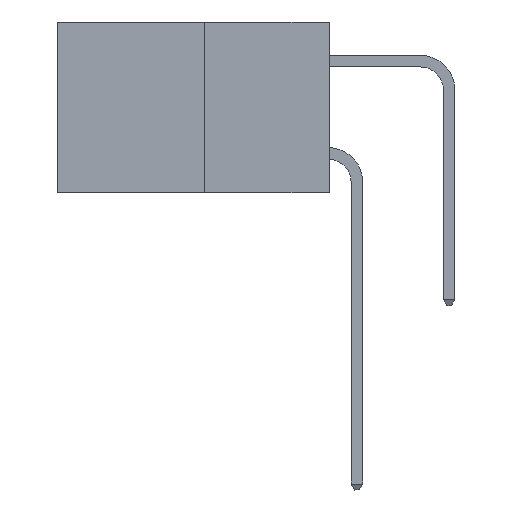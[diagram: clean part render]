
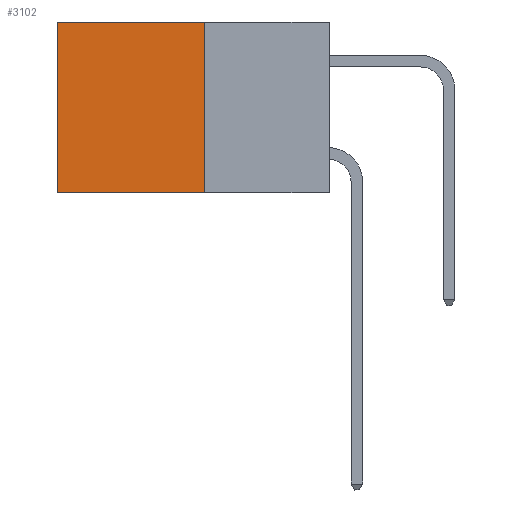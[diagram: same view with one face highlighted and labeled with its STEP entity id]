
A CAD part, left-side view. The second image highlights one B-rep face of the part: STEP entity #3102.
In plain terms, the highlighted planar face has unit normal (-1, 0, 0).
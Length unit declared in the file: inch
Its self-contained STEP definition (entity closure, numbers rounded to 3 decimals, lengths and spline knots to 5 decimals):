
#769 = CARTESIAN_POINT ( 'NONE',  ( 0.277, 0.27, -0.37 ) ) ;
#1806 = EDGE_CURVE ( 'NONE', #21932, #14569, #10224, .T. ) ;
#1830 = CARTESIAN_POINT ( 'NONE',  ( 0.277, 0.59, -0.37 ) ) ;
#2989 = EDGE_CURVE ( 'NONE', #21932, #9261, #9326, .T. ) ;
#3102 = ADVANCED_FACE ( 'NONE', ( #20293 ), #15326, .F. ) ;
#3221 = LINE ( 'NONE', #1830, #3775 ) ;
#3611 = DIRECTION ( 'NONE',  ( 0., 0., -1. ) ) ;
#3775 = VECTOR ( 'NONE', #3611, 39.37008 ) ;
#4475 = DIRECTION ( 'NONE',  ( 0., 0., -1. ) ) ;
#5391 = DIRECTION ( 'NONE',  ( 0., 0., -1. ) ) ;
#5444 = CARTESIAN_POINT ( 'NONE',  ( 0.277, 0.27, -0.37 ) ) ;
#5458 = VECTOR ( 'NONE', #4475, 39.37008 ) ;
#6815 = DIRECTION ( 'NONE',  ( 1., 0., 0. ) ) ;
#7216 = EDGE_CURVE ( 'NONE', #14569, #18405, #9170, .T. ) ;
#7908 = ORIENTED_EDGE ( 'NONE', *, *, #2989, .T. ) ;
#8544 = CARTESIAN_POINT ( 'NONE',  ( 0.277, 0.59, 0. ) ) ;
#9170 = LINE ( 'NONE', #17642, #22338 ) ;
#9196 = ORIENTED_EDGE ( 'NONE', *, *, #16429, .T. ) ;
#9261 = VERTEX_POINT ( 'NONE', #8544 ) ;
#9326 = LINE ( 'NONE', #16064, #23033 ) ;
#10224 = LINE ( 'NONE', #5444, #5458 ) ;
#13154 = CARTESIAN_POINT ( 'NONE',  ( 0.277, 0.27, 0. ) ) ;
#14569 = VERTEX_POINT ( 'NONE', #17358 ) ;
#15326 = PLANE ( 'NONE',  #16051 ) ;
#15987 = DIRECTION ( 'NONE',  ( 0., 1., 0. ) ) ;
#16051 = AXIS2_PLACEMENT_3D ( 'NONE', #769, #6815, #5391 ) ;
#16064 = CARTESIAN_POINT ( 'NONE',  ( 0.277, 0.27, 0. ) ) ;
#16429 = EDGE_CURVE ( 'NONE', #9261, #18405, #3221, .T. ) ;
#17358 = CARTESIAN_POINT ( 'NONE',  ( 0.277, 0.27, -0.37 ) ) ;
#17642 = CARTESIAN_POINT ( 'NONE',  ( 0.277, 0.27, -0.37 ) ) ;
#17667 = DIRECTION ( 'NONE',  ( 0., 1., 0. ) ) ;
#18405 = VERTEX_POINT ( 'NONE', #18869 ) ;
#18869 = CARTESIAN_POINT ( 'NONE',  ( 0.277, 0.59, -0.37 ) ) ;
#20293 = FACE_OUTER_BOUND ( 'NONE', #21726, .T. ) ;
#20826 = ORIENTED_EDGE ( 'NONE', *, *, #1806, .F. ) ;
#21726 = EDGE_LOOP ( 'NONE', ( #9196, #22639, #20826, #7908 ) ) ;
#21932 = VERTEX_POINT ( 'NONE', #13154 ) ;
#22338 = VECTOR ( 'NONE', #17667, 39.37008 ) ;
#22639 = ORIENTED_EDGE ( 'NONE', *, *, #7216, .F. ) ;
#23033 = VECTOR ( 'NONE', #15987, 39.37008 ) ;
